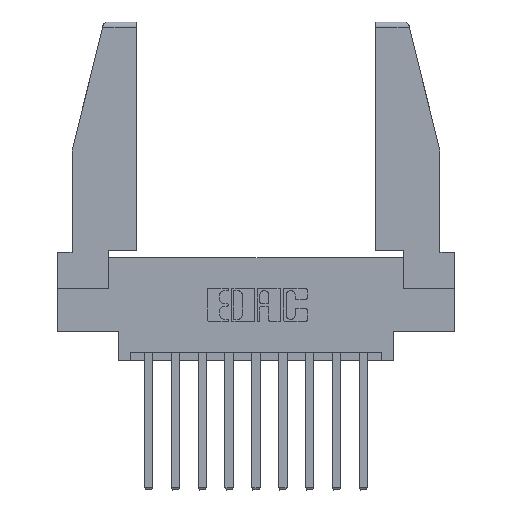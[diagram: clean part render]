
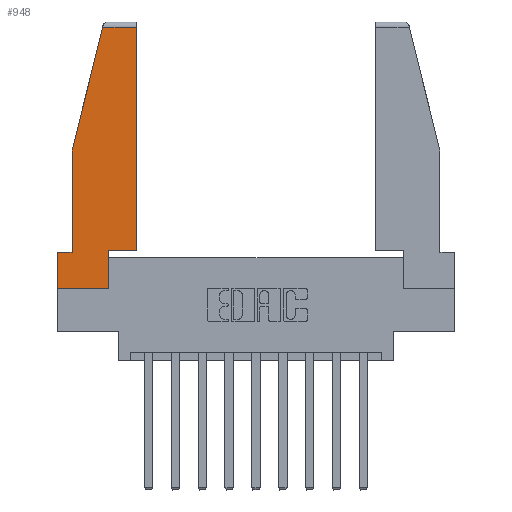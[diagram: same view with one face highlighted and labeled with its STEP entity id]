
A CAD part, top view. The second image highlights one B-rep face of the part: STEP entity #948.
In plain terms, the highlighted planar face has unit normal (0, 0, 1).
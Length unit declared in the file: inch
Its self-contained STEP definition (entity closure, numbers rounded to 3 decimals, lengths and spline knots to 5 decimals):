
#349 = DIRECTION ( 'NONE',  ( -0.239, -0.971, 0. ) ) ;
#819 = EDGE_CURVE ( 'NONE', #13351, #3194, #11995, .T. ) ;
#948 = ADVANCED_FACE ( 'NONE', ( #6731 ), #8138, .T. ) ;
#1490 = VECTOR ( 'NONE', #12736, 39.37008 ) ;
#1686 = VERTEX_POINT ( 'NONE', #2474 ) ;
#1842 = DIRECTION ( 'NONE',  ( 0., 0., 1. ) ) ;
#1926 = VERTEX_POINT ( 'NONE', #2889 ) ;
#1950 = VECTOR ( 'NONE', #13670, 39.37008 ) ;
#2386 = EDGE_CURVE ( 'NONE', #1926, #9012, #10602, .T. ) ;
#2467 = VERTEX_POINT ( 'NONE', #3375 ) ;
#2474 = CARTESIAN_POINT ( 'NONE',  ( 0.297, 0.223, 0. ) ) ;
#2529 = EDGE_CURVE ( 'NONE', #5686, #7832, #3835, .T. ) ;
#2715 = CARTESIAN_POINT ( 'NONE',  ( 0.086, 0.8, 0. ) ) ;
#2754 = CARTESIAN_POINT ( 'NONE',  ( 0.461, 1.52, 0. ) ) ;
#2889 = CARTESIAN_POINT ( 'NONE',  ( 0., 0.21, 0. ) ) ;
#3001 = LINE ( 'NONE', #7108, #5320 ) ;
#3163 = EDGE_CURVE ( 'NONE', #2467, #1686, #3001, .T. ) ;
#3194 = VERTEX_POINT ( 'NONE', #2754 ) ;
#3323 = DIRECTION ( 'NONE',  ( 0., -1., 0. ) ) ;
#3375 = CARTESIAN_POINT ( 'NONE',  ( 0.297, 0., 0. ) ) ;
#3617 = ORIENTED_EDGE ( 'NONE', *, *, #8912, .T. ) ;
#3648 = CARTESIAN_POINT ( 'NONE',  ( 0., 0., 0. ) ) ;
#3835 = LINE ( 'NONE', #5555, #5497 ) ;
#4179 = LINE ( 'NONE', #9564, #1490 ) ;
#4319 = ORIENTED_EDGE ( 'NONE', *, *, #819, .T. ) ;
#4379 = EDGE_CURVE ( 'NONE', #3194, #5686, #11363, .T. ) ;
#4645 = EDGE_LOOP ( 'NONE', ( #4319, #8075, #7016, #7494, #3617, #10503, #9376, #6347, #9831 ) ) ;
#4859 = DIRECTION ( 'NONE',  ( 1., 0., 0. ) ) ;
#5222 = VECTOR ( 'NONE', #6381, 39.37008 ) ;
#5320 = VECTOR ( 'NONE', #11137, 39.37008 ) ;
#5497 = VECTOR ( 'NONE', #349, 39.37008 ) ;
#5555 = CARTESIAN_POINT ( 'NONE',  ( 0.271, 1.55, 0. ) ) ;
#5686 = VERTEX_POINT ( 'NONE', #10727 ) ;
#6037 = EDGE_CURVE ( 'NONE', #7832, #11269, #12642, .T. ) ;
#6102 = VECTOR ( 'NONE', #12067, 39.37008 ) ;
#6347 = ORIENTED_EDGE ( 'NONE', *, *, #3163, .T. ) ;
#6381 = DIRECTION ( 'NONE',  ( -1., 0., 0. ) ) ;
#6731 = FACE_OUTER_BOUND ( 'NONE', #4645, .T. ) ;
#7016 = ORIENTED_EDGE ( 'NONE', *, *, #2529, .T. ) ;
#7108 = CARTESIAN_POINT ( 'NONE',  ( 0.297, 0., 0. ) ) ;
#7237 = CARTESIAN_POINT ( 'NONE',  ( 0., 1.52, 0. ) ) ;
#7494 = ORIENTED_EDGE ( 'NONE', *, *, #6037, .T. ) ;
#7832 = VERTEX_POINT ( 'NONE', #2715 ) ;
#7999 = LINE ( 'NONE', #8539, #5222 ) ;
#8075 = ORIENTED_EDGE ( 'NONE', *, *, #4379, .T. ) ;
#8138 = PLANE ( 'NONE',  #12379 ) ;
#8539 = CARTESIAN_POINT ( 'NONE',  ( 0., 0.21, 0. ) ) ;
#8912 = EDGE_CURVE ( 'NONE', #11269, #1926, #7999, .T. ) ;
#9012 = VERTEX_POINT ( 'NONE', #11745 ) ;
#9231 = DIRECTION ( 'NONE',  ( 1., 0., 0. ) ) ;
#9376 = ORIENTED_EDGE ( 'NONE', *, *, #12935, .T. ) ;
#9564 = CARTESIAN_POINT ( 'NONE',  ( 0.297, 0.223, 0. ) ) ;
#9571 = CARTESIAN_POINT ( 'NONE',  ( 0.461, 0.223, 0. ) ) ;
#9764 = CARTESIAN_POINT ( 'NONE',  ( 0., 0.21, 0. ) ) ;
#9831 = ORIENTED_EDGE ( 'NONE', *, *, #10713, .T. ) ;
#10503 = ORIENTED_EDGE ( 'NONE', *, *, #2386, .T. ) ;
#10602 = LINE ( 'NONE', #9764, #11885 ) ;
#10692 = VECTOR ( 'NONE', #12548, 39.37008 ) ;
#10713 = EDGE_CURVE ( 'NONE', #1686, #13351, #4179, .T. ) ;
#10727 = CARTESIAN_POINT ( 'NONE',  ( 0.2636, 1.52, 0. ) ) ;
#11030 = CARTESIAN_POINT ( 'NONE',  ( 0.461, 0.223, 0. ) ) ;
#11137 = DIRECTION ( 'NONE',  ( 0., 1., 0. ) ) ;
#11269 = VERTEX_POINT ( 'NONE', #13128 ) ;
#11363 = LINE ( 'NONE', #7237, #1950 ) ;
#11745 = CARTESIAN_POINT ( 'NONE',  ( 0., 0., 0. ) ) ;
#11885 = VECTOR ( 'NONE', #3323, 39.37008 ) ;
#11995 = LINE ( 'NONE', #11030, #6102 ) ;
#12067 = DIRECTION ( 'NONE',  ( 0., 1., 0. ) ) ;
#12167 = CARTESIAN_POINT ( 'NONE',  ( 0., 0., 0. ) ) ;
#12379 = AXIS2_PLACEMENT_3D ( 'NONE', #12167, #1842, #9231 ) ;
#12395 = VECTOR ( 'NONE', #4859, 39.37008 ) ;
#12510 = CARTESIAN_POINT ( 'NONE',  ( 0.086, 0.8, 0. ) ) ;
#12548 = DIRECTION ( 'NONE',  ( 0., -1., 0. ) ) ;
#12642 = LINE ( 'NONE', #12510, #10692 ) ;
#12736 = DIRECTION ( 'NONE',  ( 1., 0., 0. ) ) ;
#12935 = EDGE_CURVE ( 'NONE', #9012, #2467, #13221, .T. ) ;
#13128 = CARTESIAN_POINT ( 'NONE',  ( 0.086, 0.21, 0. ) ) ;
#13221 = LINE ( 'NONE', #3648, #12395 ) ;
#13351 = VERTEX_POINT ( 'NONE', #9571 ) ;
#13670 = DIRECTION ( 'NONE',  ( -1., 0., 0. ) ) ;
